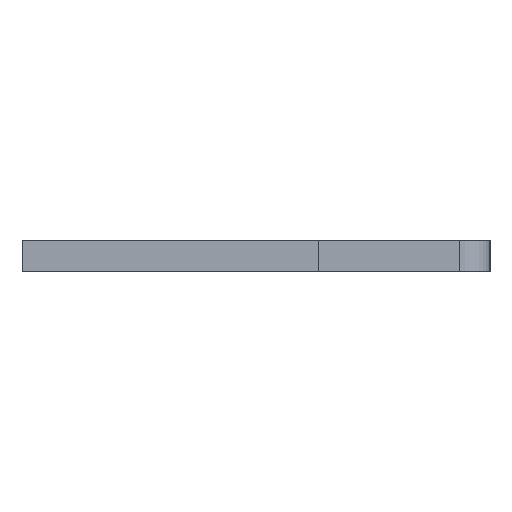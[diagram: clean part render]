
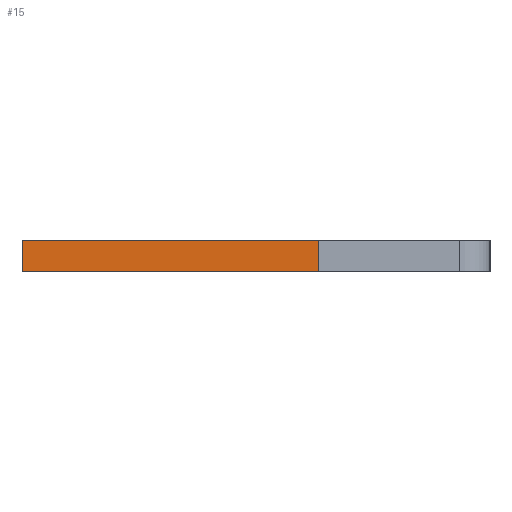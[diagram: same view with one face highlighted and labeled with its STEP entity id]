
A CAD part, left-side view. The second image highlights one B-rep face of the part: STEP entity #15.
In plain terms, the highlighted face is planar.
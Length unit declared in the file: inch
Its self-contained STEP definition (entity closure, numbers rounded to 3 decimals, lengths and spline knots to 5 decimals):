
#15 = ADVANCED_FACE ( 'NONE', ( #1188 ), #978, .F. ) ;
#61 = LINE ( 'NONE', #678, #292 ) ;
#118 = AXIS2_PLACEMENT_3D ( 'NONE', #358, #1515, #1236 ) ;
#131 = CARTESIAN_POINT ( 'NONE',  ( 0.01, 0.15, -0.04 ) ) ;
#137 = DIRECTION ( 'NONE',  ( -1., 0., 0. ) ) ;
#171 = VERTEX_POINT ( 'NONE', #738 ) ;
#256 = CARTESIAN_POINT ( 'NONE',  ( 0.01, -0.04, -0.04 ) ) ;
#285 = CARTESIAN_POINT ( 'NONE',  ( -0.01, 0.15, -0.04 ) ) ;
#292 = VECTOR ( 'NONE', #315, 39.37008 ) ;
#315 = DIRECTION ( 'NONE',  ( -1., 0., 0. ) ) ;
#358 = CARTESIAN_POINT ( 'NONE',  ( 0.01, 0.15, -0.04 ) ) ;
#373 = EDGE_CURVE ( 'NONE', #960, #171, #1174, .T. ) ;
#407 = EDGE_CURVE ( 'NONE', #960, #1278, #966, .T. ) ;
#409 = DIRECTION ( 'NONE',  ( 0., 1., 0. ) ) ;
#446 = CARTESIAN_POINT ( 'NONE',  ( 0.01, -0.04, -0.04 ) ) ;
#660 = LINE ( 'NONE', #285, #685 ) ;
#678 = CARTESIAN_POINT ( 'NONE',  ( 0.01, 0.15, -0.04 ) ) ;
#685 = VECTOR ( 'NONE', #409, 39.37008 ) ;
#722 = ORIENTED_EDGE ( 'NONE', *, *, #407, .T. ) ;
#738 = CARTESIAN_POINT ( 'NONE',  ( 0.01, 0.15, -0.04 ) ) ;
#766 = VERTEX_POINT ( 'NONE', #1181 ) ;
#825 = EDGE_CURVE ( 'NONE', #1278, #766, #660, .T. ) ;
#826 = ORIENTED_EDGE ( 'NONE', *, *, #373, .F. ) ;
#885 = EDGE_LOOP ( 'NONE', ( #1025, #1602, #826, #722 ) ) ;
#960 = VERTEX_POINT ( 'NONE', #446 ) ;
#966 = LINE ( 'NONE', #256, #1386 ) ;
#978 = PLANE ( 'NONE',  #118 ) ;
#1025 = ORIENTED_EDGE ( 'NONE', *, *, #825, .T. ) ;
#1089 = CARTESIAN_POINT ( 'NONE',  ( -0.01, -0.04, -0.04 ) ) ;
#1095 = VECTOR ( 'NONE', #1522, 39.37008 ) ;
#1174 = LINE ( 'NONE', #131, #1095 ) ;
#1181 = CARTESIAN_POINT ( 'NONE',  ( -0.01, 0.15, -0.04 ) ) ;
#1188 = FACE_OUTER_BOUND ( 'NONE', #885, .T. ) ;
#1236 = DIRECTION ( 'NONE',  ( 1., 0., 0. ) ) ;
#1257 = EDGE_CURVE ( 'NONE', #171, #766, #61, .T. ) ;
#1278 = VERTEX_POINT ( 'NONE', #1089 ) ;
#1386 = VECTOR ( 'NONE', #137, 39.37008 ) ;
#1515 = DIRECTION ( 'NONE',  ( 0., 0., 1. ) ) ;
#1522 = DIRECTION ( 'NONE',  ( 0., 1., 0. ) ) ;
#1602 = ORIENTED_EDGE ( 'NONE', *, *, #1257, .F. ) ;
